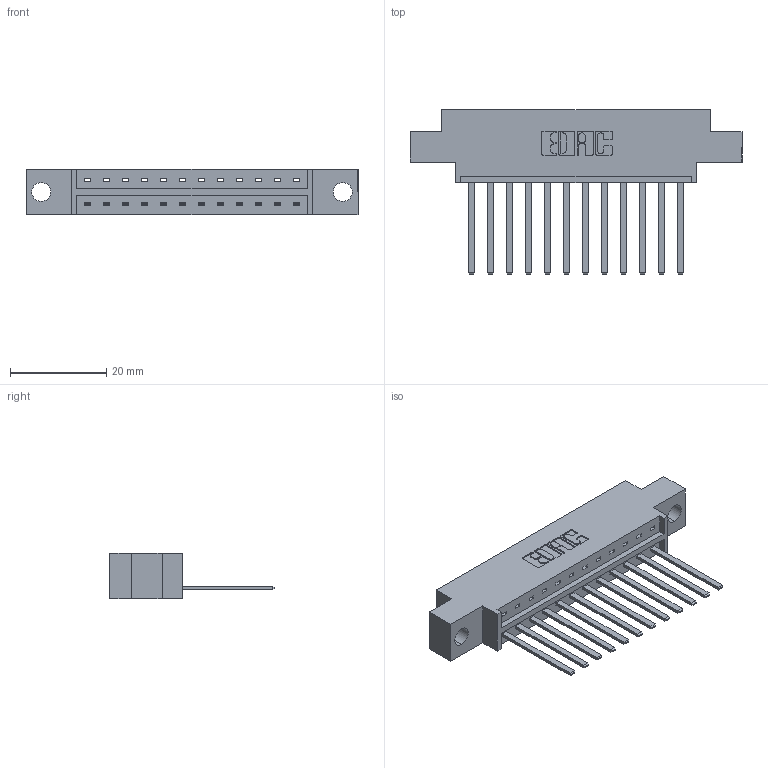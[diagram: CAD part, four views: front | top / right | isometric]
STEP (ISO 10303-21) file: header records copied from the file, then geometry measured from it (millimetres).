
FILE_DESCRIPTION (( 'STEP AP203' ), '1' );
FILE_NAME ('833-012-544-604.STEP', '2020-05-30T22:26:33', ( '' ), ( '' ), 'SwSTEP 2.0', 'SolidWorks 2020', '' );
FILE_SCHEMA (( 'CONFIG_CONTROL_DESIGN' ));
Length unit declared in the file: inch
Products named in the file (3): 833-012-544-604; 345-292-001_345-293-144; 833 Part_Offset - .156 Dia - TH
Assembly tree (13 placements, depth 2):
  833-012-544-604
    833 Part_Offset - .156 Dia - TH
    345-292-001_345-293-144  x12
Bounding box: 69.09 x 34.3 x 9.4 mm (x, y, z)
Volume: 6517.5 mm3; surface area: 7300.7 mm2
Topology: 13 solids, 13 shells, 742 faces, 2219 edges, 1462 vertices
Faces by surface type: plane 530, cylinder 212
Entity records: 11167 total; most frequent: CARTESIAN_POINT 1938, ORIENTED_EDGE 1886, DIRECTION 1691, EDGE_CURVE 943, LINE 819, VECTOR 819, VERTEX_POINT 626, AXIS2_PLACEMENT_3D 436
